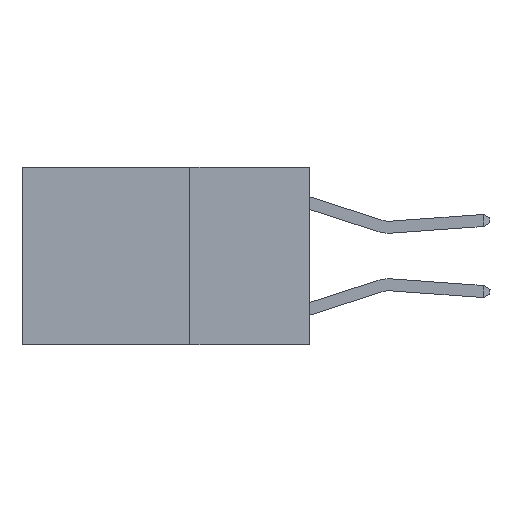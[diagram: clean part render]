
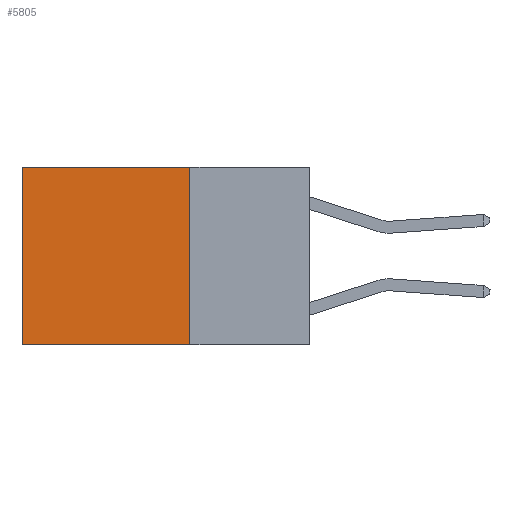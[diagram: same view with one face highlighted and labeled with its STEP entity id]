
A CAD part, left-side view. The second image highlights one B-rep face of the part: STEP entity #5805.
In plain terms, the highlighted planar face has unit normal (-1, 0, 0).
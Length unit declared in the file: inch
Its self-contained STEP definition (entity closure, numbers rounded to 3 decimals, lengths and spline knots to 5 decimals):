
#251 = ORIENTED_EDGE ( 'NONE', *, *, #21332, .T. ) ;
#794 = DIRECTION ( 'NONE',  ( 1., 0., 0. ) ) ;
#1020 = CARTESIAN_POINT ( 'NONE',  ( 0.2625, 0.6, 0. ) ) ;
#2185 = EDGE_CURVE ( 'NONE', #21711, #22103, #18375, .T. ) ;
#2542 = DIRECTION ( 'NONE',  ( 0., 0., -1. ) ) ;
#2636 = ORIENTED_EDGE ( 'NONE', *, *, #23723, .F. ) ;
#4482 = VECTOR ( 'NONE', #25781, 39.37008 ) ;
#5024 = VECTOR ( 'NONE', #15236, 39.37008 ) ;
#5288 = VERTEX_POINT ( 'NONE', #8197 ) ;
#5441 = PLANE ( 'NONE',  #16765 ) ;
#5805 = ADVANCED_FACE ( 'NONE', ( #20867 ), #5441, .F. ) ;
#8197 = CARTESIAN_POINT ( 'NONE',  ( 0.2625, 0.25, 0. ) ) ;
#8919 = LINE ( 'NONE', #20516, #14596 ) ;
#12635 = CARTESIAN_POINT ( 'NONE',  ( 0.2625, 0.25, 0. ) ) ;
#14596 = VECTOR ( 'NONE', #18589, 39.37008 ) ;
#14773 = LINE ( 'NONE', #24549, #21562 ) ;
#15236 = DIRECTION ( 'NONE',  ( 0., 1., 0. ) ) ;
#16765 = AXIS2_PLACEMENT_3D ( 'NONE', #22796, #794, #20387 ) ;
#18375 = LINE ( 'NONE', #22880, #4482 ) ;
#18589 = DIRECTION ( 'NONE',  ( 0., 1., 0. ) ) ;
#20387 = DIRECTION ( 'NONE',  ( 0., 0., -1. ) ) ;
#20516 = CARTESIAN_POINT ( 'NONE',  ( 0.2625, 0.25, -0.37 ) ) ;
#20867 = FACE_OUTER_BOUND ( 'NONE', #26553, .T. ) ;
#21332 = EDGE_CURVE ( 'NONE', #5288, #21711, #26782, .T. ) ;
#21562 = VECTOR ( 'NONE', #2542, 39.37008 ) ;
#21711 = VERTEX_POINT ( 'NONE', #1020 ) ;
#22103 = VERTEX_POINT ( 'NONE', #25216 ) ;
#22796 = CARTESIAN_POINT ( 'NONE',  ( 0.2625, 0.25, 0. ) ) ;
#22880 = CARTESIAN_POINT ( 'NONE',  ( 0.2625, 0.6, 0. ) ) ;
#23484 = VERTEX_POINT ( 'NONE', #26500 ) ;
#23723 = EDGE_CURVE ( 'NONE', #5288, #23484, #14773, .T. ) ;
#24326 = ORIENTED_EDGE ( 'NONE', *, *, #2185, .T. ) ;
#24549 = CARTESIAN_POINT ( 'NONE',  ( 0.2625, 0.25, 0. ) ) ;
#25216 = CARTESIAN_POINT ( 'NONE',  ( 0.2625, 0.6, -0.37 ) ) ;
#25781 = DIRECTION ( 'NONE',  ( 0., 0., -1. ) ) ;
#26500 = CARTESIAN_POINT ( 'NONE',  ( 0.2625, 0.25, -0.37 ) ) ;
#26553 = EDGE_LOOP ( 'NONE', ( #24326, #30699, #2636, #251 ) ) ;
#26782 = LINE ( 'NONE', #12635, #5024 ) ;
#28747 = EDGE_CURVE ( 'NONE', #23484, #22103, #8919, .T. ) ;
#30699 = ORIENTED_EDGE ( 'NONE', *, *, #28747, .F. ) ;
